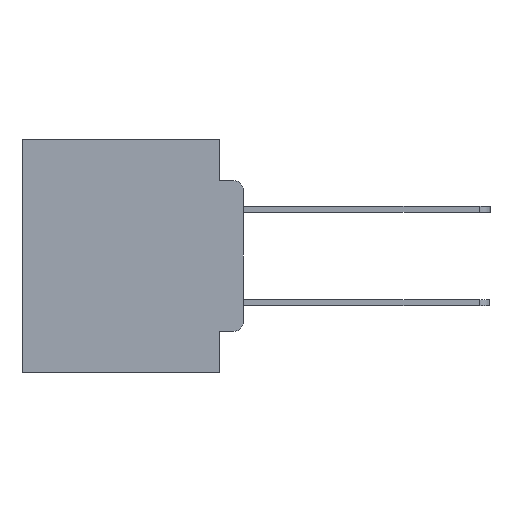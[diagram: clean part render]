
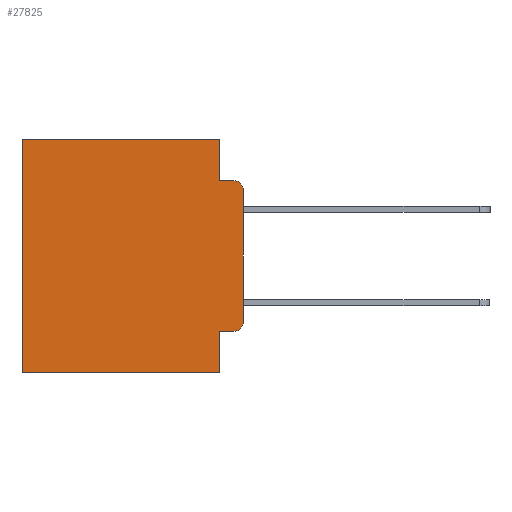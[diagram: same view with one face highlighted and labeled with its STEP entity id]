
A CAD part, left-side view. The second image highlights one B-rep face of the part: STEP entity #27825.
In plain terms, the highlighted planar face has unit normal (-1, 0, 0).
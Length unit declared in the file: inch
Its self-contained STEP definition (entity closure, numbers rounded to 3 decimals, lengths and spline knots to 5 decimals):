
#396 = LINE ( 'NONE', #20789, #6047 ) ;
#478 = DIRECTION ( 'NONE',  ( 1., 0., 0. ) ) ;
#492 = VERTEX_POINT ( 'NONE', #26113 ) ;
#947 = CARTESIAN_POINT ( 'NONE',  ( 0.298, 0.473, 0. ) ) ;
#960 = ORIENTED_EDGE ( 'NONE', *, *, #2682, .T. ) ;
#1322 = LINE ( 'NONE', #26560, #13022 ) ;
#1474 = DIRECTION ( 'NONE',  ( 0., 0., -1. ) ) ;
#2061 = VERTEX_POINT ( 'NONE', #947 ) ;
#2199 = CARTESIAN_POINT ( 'NONE',  ( 0.298, 0.051, 0. ) ) ;
#2485 = DIRECTION ( 'NONE',  ( 0., -1., 0. ) ) ;
#2519 = CIRCLE ( 'NONE', #18250, 0.02 ) ;
#2521 = ORIENTED_EDGE ( 'NONE', *, *, #16610, .T. ) ;
#2527 = DIRECTION ( 'NONE',  ( -1., 0., 0. ) ) ;
#2609 = CARTESIAN_POINT ( 'NONE',  ( 0.298, 0.051, -0.4115 ) ) ;
#2682 = EDGE_CURVE ( 'NONE', #19272, #23825, #2519, .T. ) ;
#2887 = ORIENTED_EDGE ( 'NONE', *, *, #29267, .F. ) ;
#3360 = LINE ( 'NONE', #25812, #5596 ) ;
#3570 = LINE ( 'NONE', #2199, #15085 ) ;
#4026 = CARTESIAN_POINT ( 'NONE',  ( 0.298, 0., -0.3915 ) ) ;
#4520 = DIRECTION ( 'NONE',  ( 0., 0., -1. ) ) ;
#5119 = ORIENTED_EDGE ( 'NONE', *, *, #7407, .F. ) ;
#5241 = VECTOR ( 'NONE', #13332, 39.37008 ) ;
#5596 = VECTOR ( 'NONE', #12187, 39.37008 ) ;
#6047 = VECTOR ( 'NONE', #2485, 39.37008 ) ;
#6901 = ORIENTED_EDGE ( 'NONE', *, *, #10022, .F. ) ;
#7101 = EDGE_CURVE ( 'NONE', #492, #2061, #29396, .T. ) ;
#7407 = EDGE_CURVE ( 'NONE', #18035, #23825, #3360, .T. ) ;
#7442 = CARTESIAN_POINT ( 'NONE',  ( 0.298, 0.473, -0.5 ) ) ;
#8931 = EDGE_CURVE ( 'NONE', #492, #18035, #15879, .T. ) ;
#9314 = DIRECTION ( 'NONE',  ( 0., 0., -1. ) ) ;
#10022 = EDGE_CURVE ( 'NONE', #17205, #16105, #16170, .T. ) ;
#10061 = VECTOR ( 'NONE', #14337, 39.37008 ) ;
#10812 = CARTESIAN_POINT ( 'NONE',  ( 0.298, 0.02, -0.4115 ) ) ;
#11020 = CARTESIAN_POINT ( 'NONE',  ( 0.298, 0., 0. ) ) ;
#12187 = DIRECTION ( 'NONE',  ( 0., -1., 0. ) ) ;
#12555 = DIRECTION ( 'NONE',  ( -1., 0., 0. ) ) ;
#13022 = VECTOR ( 'NONE', #21960, 39.37008 ) ;
#13332 = DIRECTION ( 'NONE',  ( 0., 1., 0. ) ) ;
#13582 = EDGE_CURVE ( 'NONE', #2061, #16105, #1322, .T. ) ;
#13906 = AXIS2_PLACEMENT_3D ( 'NONE', #14462, #478, #16752 ) ;
#13911 = CARTESIAN_POINT ( 'NONE',  ( 0.298, 0.051, -0.5 ) ) ;
#14130 = VECTOR ( 'NONE', #22206, 39.37008 ) ;
#14185 = CARTESIAN_POINT ( 'NONE',  ( 0.298, 0., -0.1085 ) ) ;
#14337 = DIRECTION ( 'NONE',  ( 0., 1., 0. ) ) ;
#14430 = ORIENTED_EDGE ( 'NONE', *, *, #13582, .T. ) ;
#14462 = CARTESIAN_POINT ( 'NONE',  ( 0.298, 0., 0. ) ) ;
#14603 = CARTESIAN_POINT ( 'NONE',  ( 0.298, 0.02, -0.0885 ) ) ;
#14752 = CARTESIAN_POINT ( 'NONE',  ( 0.298, 0.051, -0.0885 ) ) ;
#14829 = ORIENTED_EDGE ( 'NONE', *, *, #15067, .F. ) ;
#15067 = EDGE_CURVE ( 'NONE', #19871, #17205, #3570, .T. ) ;
#15085 = VECTOR ( 'NONE', #4520, 39.37008 ) ;
#15141 = VECTOR ( 'NONE', #1474, 39.37008 ) ;
#15866 = ORIENTED_EDGE ( 'NONE', *, *, #8931, .F. ) ;
#15879 = LINE ( 'NONE', #28926, #15141 ) ;
#15892 = CIRCLE ( 'NONE', #24393, 0.02 ) ;
#16105 = VERTEX_POINT ( 'NONE', #7442 ) ;
#16170 = LINE ( 'NONE', #27903, #10061 ) ;
#16610 = EDGE_CURVE ( 'NONE', #19871, #20817, #396, .T. ) ;
#16752 = DIRECTION ( 'NONE',  ( 0., 0., -1. ) ) ;
#17205 = VERTEX_POINT ( 'NONE', #13911 ) ;
#17321 = EDGE_LOOP ( 'NONE', ( #2887, #960, #5119, #15866, #27227, #14430, #6901, #14829, #2521, #25505 ) ) ;
#18027 = CARTESIAN_POINT ( 'NONE',  ( 0.298, 0.02, -0.1085 ) ) ;
#18035 = VERTEX_POINT ( 'NONE', #14752 ) ;
#18140 = EDGE_CURVE ( 'NONE', #20817, #25577, #15892, .T. ) ;
#18250 = AXIS2_PLACEMENT_3D ( 'NONE', #18027, #2527, #9314 ) ;
#19272 = VERTEX_POINT ( 'NONE', #14185 ) ;
#19871 = VERTEX_POINT ( 'NONE', #2609 ) ;
#20789 = CARTESIAN_POINT ( 'NONE',  ( 0.298, 0.051, -0.4115 ) ) ;
#20817 = VERTEX_POINT ( 'NONE', #10812 ) ;
#21569 = LINE ( 'NONE', #24414, #14130 ) ;
#21960 = DIRECTION ( 'NONE',  ( 0., 0., -1. ) ) ;
#22206 = DIRECTION ( 'NONE',  ( 0., 0., -1. ) ) ;
#23493 = PLANE ( 'NONE',  #13906 ) ;
#23825 = VERTEX_POINT ( 'NONE', #14603 ) ;
#24393 = AXIS2_PLACEMENT_3D ( 'NONE', #26174, #12555, #28390 ) ;
#24414 = CARTESIAN_POINT ( 'NONE',  ( 0.298, 0., 0. ) ) ;
#25250 = FACE_OUTER_BOUND ( 'NONE', #17321, .T. ) ;
#25505 = ORIENTED_EDGE ( 'NONE', *, *, #18140, .T. ) ;
#25577 = VERTEX_POINT ( 'NONE', #4026 ) ;
#25812 = CARTESIAN_POINT ( 'NONE',  ( 0.298, 0.051, -0.0885 ) ) ;
#26113 = CARTESIAN_POINT ( 'NONE',  ( 0.298, 0.051, 0. ) ) ;
#26174 = CARTESIAN_POINT ( 'NONE',  ( 0.298, 0.02, -0.3915 ) ) ;
#26560 = CARTESIAN_POINT ( 'NONE',  ( 0.298, 0.473, 0. ) ) ;
#27227 = ORIENTED_EDGE ( 'NONE', *, *, #7101, .T. ) ;
#27825 = ADVANCED_FACE ( 'NONE', ( #25250 ), #23493, .F. ) ;
#27903 = CARTESIAN_POINT ( 'NONE',  ( 0.298, 0., -0.5 ) ) ;
#28390 = DIRECTION ( 'NONE',  ( 0., 0., -1. ) ) ;
#28926 = CARTESIAN_POINT ( 'NONE',  ( 0.298, 0.051, 0. ) ) ;
#29267 = EDGE_CURVE ( 'NONE', #19272, #25577, #21569, .T. ) ;
#29396 = LINE ( 'NONE', #11020, #5241 ) ;
